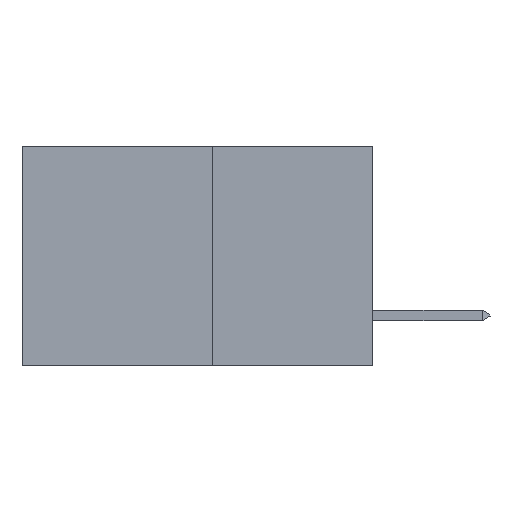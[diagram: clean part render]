
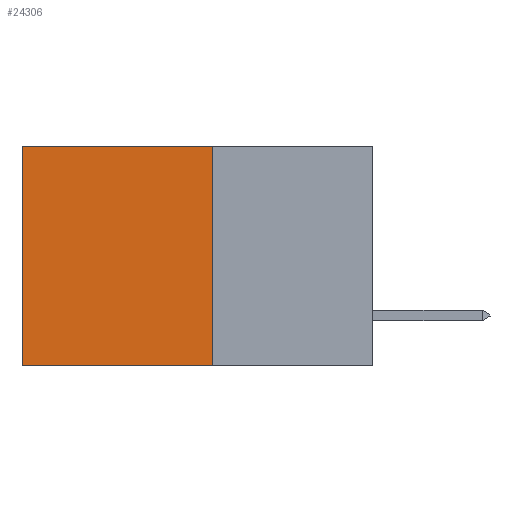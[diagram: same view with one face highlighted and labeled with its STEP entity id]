
A CAD part, left-side view. The second image highlights one B-rep face of the part: STEP entity #24306.
In plain terms, the highlighted planar face has unit normal (-1, 0, 0).
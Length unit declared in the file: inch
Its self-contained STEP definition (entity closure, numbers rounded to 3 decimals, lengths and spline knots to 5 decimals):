
#144 = CARTESIAN_POINT ( 'NONE',  ( 0.277, 0.27, -0.37 ) ) ;
#1467 = ORIENTED_EDGE ( 'NONE', *, *, #25660, .T. ) ;
#1560 = VERTEX_POINT ( 'NONE', #25924 ) ;
#1871 = EDGE_CURVE ( 'NONE', #1560, #3470, #31817, .T. ) ;
#2627 = CARTESIAN_POINT ( 'NONE',  ( 0.277, 0.27, 0. ) ) ;
#2758 = CARTESIAN_POINT ( 'NONE',  ( 0.277, 0.59, -0.37 ) ) ;
#3417 = CARTESIAN_POINT ( 'NONE',  ( 0.277, 0.27, -0.37 ) ) ;
#3470 = VERTEX_POINT ( 'NONE', #144 ) ;
#4662 = CARTESIAN_POINT ( 'NONE',  ( 0.277, 0.27, -0.37 ) ) ;
#5109 = DIRECTION ( 'NONE',  ( 0., 1., 0. ) ) ;
#5715 = DIRECTION ( 'NONE',  ( 0., 0., -1. ) ) ;
#8058 = ORIENTED_EDGE ( 'NONE', *, *, #14196, .F. ) ;
#10653 = CARTESIAN_POINT ( 'NONE',  ( 0.277, 0.59, -0.37 ) ) ;
#10963 = PLANE ( 'NONE',  #22893 ) ;
#12143 = VECTOR ( 'NONE', #14584, 39.37008 ) ;
#13142 = CARTESIAN_POINT ( 'NONE',  ( 0.277, 0.27, -0.37 ) ) ;
#13433 = DIRECTION ( 'NONE',  ( 1., 0., 0. ) ) ;
#14196 = EDGE_CURVE ( 'NONE', #3470, #22825, #18662, .T. ) ;
#14317 = VERTEX_POINT ( 'NONE', #19918 ) ;
#14584 = DIRECTION ( 'NONE',  ( 0., 1., 0. ) ) ;
#18632 = VECTOR ( 'NONE', #5109, 39.37008 ) ;
#18662 = LINE ( 'NONE', #4662, #12143 ) ;
#18743 = VECTOR ( 'NONE', #30226, 39.37008 ) ;
#19219 = EDGE_LOOP ( 'NONE', ( #1467, #8058, #27736, #29674 ) ) ;
#19415 = LINE ( 'NONE', #2627, #18632 ) ;
#19918 = CARTESIAN_POINT ( 'NONE',  ( 0.277, 0.59, 0. ) ) ;
#21009 = EDGE_CURVE ( 'NONE', #1560, #14317, #19415, .T. ) ;
#22825 = VERTEX_POINT ( 'NONE', #2758 ) ;
#22893 = AXIS2_PLACEMENT_3D ( 'NONE', #3417, #13433, #30603 ) ;
#24306 = ADVANCED_FACE ( 'NONE', ( #26143 ), #10963, .F. ) ;
#25660 = EDGE_CURVE ( 'NONE', #14317, #22825, #25720, .T. ) ;
#25720 = LINE ( 'NONE', #10653, #31469 ) ;
#25924 = CARTESIAN_POINT ( 'NONE',  ( 0.277, 0.27, 0. ) ) ;
#26143 = FACE_OUTER_BOUND ( 'NONE', #19219, .T. ) ;
#27736 = ORIENTED_EDGE ( 'NONE', *, *, #1871, .F. ) ;
#29674 = ORIENTED_EDGE ( 'NONE', *, *, #21009, .T. ) ;
#30226 = DIRECTION ( 'NONE',  ( 0., 0., -1. ) ) ;
#30603 = DIRECTION ( 'NONE',  ( 0., 0., -1. ) ) ;
#31469 = VECTOR ( 'NONE', #5715, 39.37008 ) ;
#31817 = LINE ( 'NONE', #13142, #18743 ) ;
